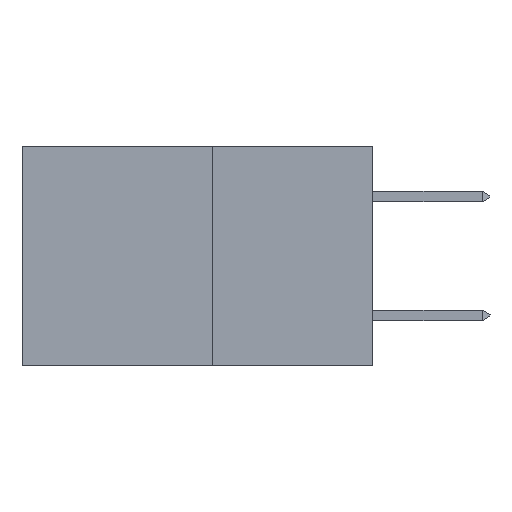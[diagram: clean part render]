
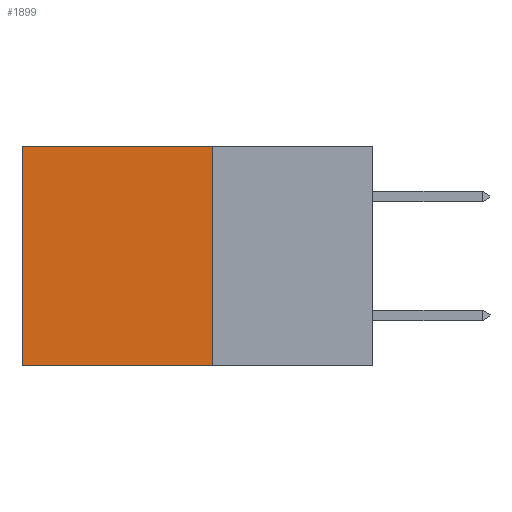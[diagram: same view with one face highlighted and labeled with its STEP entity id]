
A CAD part, left-side view. The second image highlights one B-rep face of the part: STEP entity #1899.
In plain terms, the highlighted planar face has unit normal (-1, 0, 0).
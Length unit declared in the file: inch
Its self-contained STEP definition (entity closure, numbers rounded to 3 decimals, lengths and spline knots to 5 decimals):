
#652 = VERTEX_POINT ( 'NONE', #14090 ) ;
#1606 = EDGE_CURVE ( 'NONE', #5622, #2549, #22092, .T. ) ;
#1852 = DIRECTION ( 'NONE',  ( 0., 1., 0. ) ) ;
#1899 = ADVANCED_FACE ( 'NONE', ( #6273 ), #8025, .F. ) ;
#2347 = CARTESIAN_POINT ( 'NONE',  ( 0.277, 0.27, -0.37 ) ) ;
#2549 = VERTEX_POINT ( 'NONE', #8571 ) ;
#5389 = EDGE_CURVE ( 'NONE', #12107, #2549, #27196, .T. ) ;
#5622 = VERTEX_POINT ( 'NONE', #14804 ) ;
#6273 = FACE_OUTER_BOUND ( 'NONE', #13334, .T. ) ;
#7277 = LINE ( 'NONE', #12474, #26894 ) ;
#7455 = VECTOR ( 'NONE', #14633, 39.37008 ) ;
#7679 = DIRECTION ( 'NONE',  ( 0., 0., -1. ) ) ;
#7812 = DIRECTION ( 'NONE',  ( 1., 0., 0. ) ) ;
#8025 = PLANE ( 'NONE',  #28758 ) ;
#8379 = CARTESIAN_POINT ( 'NONE',  ( 0.277, 0.27, -0.37 ) ) ;
#8571 = CARTESIAN_POINT ( 'NONE',  ( 0.277, 0.59, -0.37 ) ) ;
#11356 = ORIENTED_EDGE ( 'NONE', *, *, #23322, .F. ) ;
#12107 = VERTEX_POINT ( 'NONE', #14685 ) ;
#12474 = CARTESIAN_POINT ( 'NONE',  ( 0.277, 0.27, 0. ) ) ;
#13086 = LINE ( 'NONE', #26318, #30373 ) ;
#13334 = EDGE_LOOP ( 'NONE', ( #20718, #22151, #11356, #17830 ) ) ;
#14090 = CARTESIAN_POINT ( 'NONE',  ( 0.277, 0.27, 0. ) ) ;
#14485 = CARTESIAN_POINT ( 'NONE',  ( 0.277, 0.59, -0.37 ) ) ;
#14633 = DIRECTION ( 'NONE',  ( 0., 0., -1. ) ) ;
#14685 = CARTESIAN_POINT ( 'NONE',  ( 0.277, 0.27, -0.37 ) ) ;
#14804 = CARTESIAN_POINT ( 'NONE',  ( 0.277, 0.59, 0. ) ) ;
#17830 = ORIENTED_EDGE ( 'NONE', *, *, #22879, .T. ) ;
#20718 = ORIENTED_EDGE ( 'NONE', *, *, #1606, .T. ) ;
#22092 = LINE ( 'NONE', #14485, #7455 ) ;
#22151 = ORIENTED_EDGE ( 'NONE', *, *, #5389, .F. ) ;
#22220 = VECTOR ( 'NONE', #1852, 39.37008 ) ;
#22879 = EDGE_CURVE ( 'NONE', #652, #5622, #7277, .T. ) ;
#23322 = EDGE_CURVE ( 'NONE', #652, #12107, #13086, .T. ) ;
#26318 = CARTESIAN_POINT ( 'NONE',  ( 0.277, 0.27, -0.37 ) ) ;
#26894 = VECTOR ( 'NONE', #29668, 39.37008 ) ;
#27196 = LINE ( 'NONE', #2347, #22220 ) ;
#28758 = AXIS2_PLACEMENT_3D ( 'NONE', #8379, #7812, #7679 ) ;
#28796 = DIRECTION ( 'NONE',  ( 0., 0., -1. ) ) ;
#29668 = DIRECTION ( 'NONE',  ( 0., 1., 0. ) ) ;
#30373 = VECTOR ( 'NONE', #28796, 39.37008 ) ;
